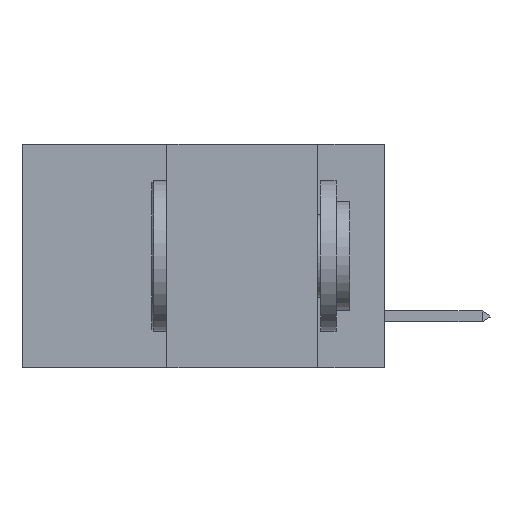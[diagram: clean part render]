
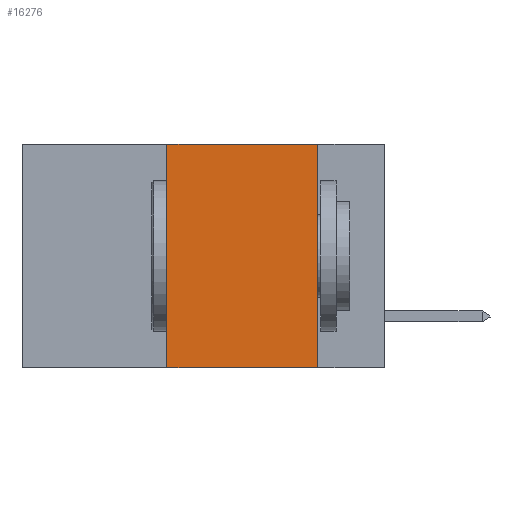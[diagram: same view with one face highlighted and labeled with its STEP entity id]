
A CAD part, left-side view. The second image highlights one B-rep face of the part: STEP entity #16276.
In plain terms, the highlighted planar face has unit normal (-1, 0, 0).
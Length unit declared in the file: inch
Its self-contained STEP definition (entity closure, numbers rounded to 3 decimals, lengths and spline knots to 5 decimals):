
#603 = CARTESIAN_POINT ( 'NONE',  ( 0., 0.11, 0. ) ) ;
#1473 = VERTEX_POINT ( 'NONE', #2947 ) ;
#1647 = EDGE_LOOP ( 'NONE', ( #4496, #18987, #35427, #6102 ) ) ;
#2947 = CARTESIAN_POINT ( 'NONE',  ( 0., 0.11, -0.37 ) ) ;
#3216 = EDGE_CURVE ( 'NONE', #20529, #33800, #28356, .T. ) ;
#4496 = ORIENTED_EDGE ( 'NONE', *, *, #39340, .F. ) ;
#6102 = ORIENTED_EDGE ( 'NONE', *, *, #6333, .T. ) ;
#6333 = EDGE_CURVE ( 'NONE', #16991, #1473, #25871, .T. ) ;
#7243 = CARTESIAN_POINT ( 'NONE',  ( 0., 0.6, -0.37 ) ) ;
#9203 = EDGE_CURVE ( 'NONE', #16991, #20529, #37480, .T. ) ;
#9676 = CARTESIAN_POINT ( 'NONE',  ( 0., 0.36, 0. ) ) ;
#12551 = VECTOR ( 'NONE', #14861, 39.37008 ) ;
#14839 = DIRECTION ( 'NONE',  ( 0., -1., 0. ) ) ;
#14861 = DIRECTION ( 'NONE',  ( 0., -1., 0. ) ) ;
#16252 = DIRECTION ( 'NONE',  ( 1., 0., 0. ) ) ;
#16269 = VECTOR ( 'NONE', #14839, 39.37008 ) ;
#16276 = ADVANCED_FACE ( 'NONE', ( #42193 ), #30604, .F. ) ;
#16991 = VERTEX_POINT ( 'NONE', #44465 ) ;
#17727 = LINE ( 'NONE', #22814, #35750 ) ;
#18864 = VECTOR ( 'NONE', #21949, 39.37008 ) ;
#18987 = ORIENTED_EDGE ( 'NONE', *, *, #3216, .F. ) ;
#20529 = VERTEX_POINT ( 'NONE', #9676 ) ;
#21949 = DIRECTION ( 'NONE',  ( 0., 0., 1. ) ) ;
#22814 = CARTESIAN_POINT ( 'NONE',  ( 0., 0.11, 0. ) ) ;
#23430 = DIRECTION ( 'NONE',  ( 0., 0., -1. ) ) ;
#25871 = LINE ( 'NONE', #7243, #16269 ) ;
#26821 = CARTESIAN_POINT ( 'NONE',  ( 0., 0.36, 0. ) ) ;
#27922 = DIRECTION ( 'NONE',  ( 0., 0., -1. ) ) ;
#28356 = LINE ( 'NONE', #36275, #12551 ) ;
#30604 = PLANE ( 'NONE',  #42690 ) ;
#33800 = VERTEX_POINT ( 'NONE', #603 ) ;
#35427 = ORIENTED_EDGE ( 'NONE', *, *, #9203, .F. ) ;
#35750 = VECTOR ( 'NONE', #23430, 39.37008 ) ;
#36275 = CARTESIAN_POINT ( 'NONE',  ( 0., 0.6, 0. ) ) ;
#37480 = LINE ( 'NONE', #26821, #18864 ) ;
#37838 = CARTESIAN_POINT ( 'NONE',  ( 0., 0.6, 0. ) ) ;
#39340 = EDGE_CURVE ( 'NONE', #33800, #1473, #17727, .T. ) ;
#42193 = FACE_OUTER_BOUND ( 'NONE', #1647, .T. ) ;
#42690 = AXIS2_PLACEMENT_3D ( 'NONE', #37838, #16252, #27922 ) ;
#44465 = CARTESIAN_POINT ( 'NONE',  ( 0., 0.36, -0.37 ) ) ;
